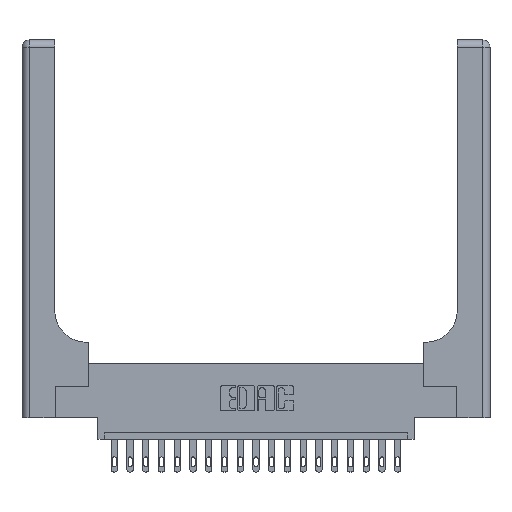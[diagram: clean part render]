
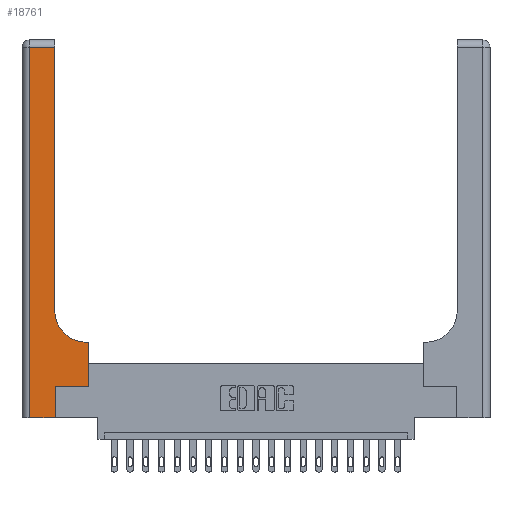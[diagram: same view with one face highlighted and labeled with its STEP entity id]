
A CAD part, top view. The second image highlights one B-rep face of the part: STEP entity #18761.
In plain terms, the highlighted planar face has unit normal (0, 0, 1).
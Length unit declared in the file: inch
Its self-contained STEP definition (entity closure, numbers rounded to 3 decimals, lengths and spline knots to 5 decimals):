
#258 = LINE ( 'NONE', #11203, #923 ) ;
#858 = CARTESIAN_POINT ( 'NONE',  ( 0.265, 0.25, 0.37 ) ) ;
#923 = VECTOR ( 'NONE', #11406, 39.37008 ) ;
#1266 = CARTESIAN_POINT ( 'NONE',  ( 0., 0., 0.37 ) ) ;
#1368 = CARTESIAN_POINT ( 'NONE',  ( 0.26, 2.94, 0.37 ) ) ;
#1375 = VECTOR ( 'NONE', #10543, 39.37008 ) ;
#1399 = LINE ( 'NONE', #14315, #11642 ) ;
#1414 = VERTEX_POINT ( 'NONE', #20177 ) ;
#1549 = VERTEX_POINT ( 'NONE', #19027 ) ;
#1613 = DIRECTION ( 'NONE',  ( 0., 1., 0. ) ) ;
#1719 = VERTEX_POINT ( 'NONE', #9852 ) ;
#1917 = CARTESIAN_POINT ( 'NONE',  ( 0.265, 0., 0.37 ) ) ;
#2539 = LINE ( 'NONE', #18473, #16022 ) ;
#2615 = VECTOR ( 'NONE', #1613, 39.37008 ) ;
#3001 = ORIENTED_EDGE ( 'NONE', *, *, #14362, .T. ) ;
#3083 = VERTEX_POINT ( 'NONE', #10987 ) ;
#3354 = EDGE_CURVE ( 'NONE', #12453, #18221, #10475, .T. ) ;
#4031 = CIRCLE ( 'NONE', #13350, 0.25 ) ;
#4135 = DIRECTION ( 'NONE',  ( -1., 0., 0. ) ) ;
#4143 = DIRECTION ( 'NONE',  ( 1., 0., 0. ) ) ;
#4725 = EDGE_CURVE ( 'NONE', #18021, #11053, #12879, .T. ) ;
#5205 = VECTOR ( 'NONE', #4135, 39.37008 ) ;
#5361 = AXIS2_PLACEMENT_3D ( 'NONE', #11034, #7587, #12482 ) ;
#7350 = CARTESIAN_POINT ( 'NONE',  ( 0., 2.94, 0.37 ) ) ;
#7587 = DIRECTION ( 'NONE',  ( 0., 0., -1. ) ) ;
#7673 = CARTESIAN_POINT ( 'NONE',  ( 0.265, 0.25, 0.37 ) ) ;
#8490 = VECTOR ( 'NONE', #19568, 39.37008 ) ;
#8946 = CARTESIAN_POINT ( 'NONE',  ( 0.265, 0., 0.37 ) ) ;
#9106 = ORIENTED_EDGE ( 'NONE', *, *, #4725, .T. ) ;
#9364 = CARTESIAN_POINT ( 'NONE',  ( 0.06, 2.94, 0.37 ) ) ;
#9852 = CARTESIAN_POINT ( 'NONE',  ( 0.06, 0., 0.37 ) ) ;
#9889 = LINE ( 'NONE', #14573, #8490 ) ;
#10297 = ORIENTED_EDGE ( 'NONE', *, *, #12374, .T. ) ;
#10475 = LINE ( 'NONE', #7350, #5205 ) ;
#10543 = DIRECTION ( 'NONE',  ( 1., 0., 0. ) ) ;
#10805 = ORIENTED_EDGE ( 'NONE', *, *, #11352, .T. ) ;
#10890 = DIRECTION ( 'NONE',  ( 0., 1., 0. ) ) ;
#10983 = VERTEX_POINT ( 'NONE', #19495 ) ;
#10987 = CARTESIAN_POINT ( 'NONE',  ( 0.51, 0.6, 0.37 ) ) ;
#11034 = CARTESIAN_POINT ( 'NONE',  ( 0., 3., 0.37 ) ) ;
#11053 = VERTEX_POINT ( 'NONE', #858 ) ;
#11203 = CARTESIAN_POINT ( 'NONE',  ( 0.528, 0.25, 0.37 ) ) ;
#11227 = LINE ( 'NONE', #7673, #15912 ) ;
#11352 = EDGE_CURVE ( 'NONE', #18221, #1719, #9889, .T. ) ;
#11406 = DIRECTION ( 'NONE',  ( 0., 1., 0. ) ) ;
#11642 = VECTOR ( 'NONE', #10890, 39.37008 ) ;
#11855 = CARTESIAN_POINT ( 'NONE',  ( 0.51, 0.85, 0.37 ) ) ;
#12374 = EDGE_CURVE ( 'NONE', #1719, #18021, #15319, .T. ) ;
#12453 = VERTEX_POINT ( 'NONE', #1368 ) ;
#12469 = DIRECTION ( 'NONE',  ( 1., 0., 0. ) ) ;
#12482 = DIRECTION ( 'NONE',  ( -1., 0., 0. ) ) ;
#12879 = LINE ( 'NONE', #1917, #2615 ) ;
#13260 = ORIENTED_EDGE ( 'NONE', *, *, #19162, .T. ) ;
#13350 = AXIS2_PLACEMENT_3D ( 'NONE', #11855, #18388, #4143 ) ;
#13750 = EDGE_CURVE ( 'NONE', #10983, #1549, #258, .T. ) ;
#13948 = EDGE_LOOP ( 'NONE', ( #20032, #19514, #10805, #10297, #9106, #3001, #17373, #16689, #13260 ) ) ;
#14315 = CARTESIAN_POINT ( 'NONE',  ( 0.26, 3., 0.37 ) ) ;
#14362 = EDGE_CURVE ( 'NONE', #11053, #10983, #11227, .T. ) ;
#14573 = CARTESIAN_POINT ( 'NONE',  ( 0.06, 3., 0.37 ) ) ;
#15319 = LINE ( 'NONE', #1266, #1375 ) ;
#15390 = PLANE ( 'NONE',  #5361 ) ;
#15912 = VECTOR ( 'NONE', #12469, 39.37008 ) ;
#16022 = VECTOR ( 'NONE', #20422, 39.37008 ) ;
#16689 = ORIENTED_EDGE ( 'NONE', *, *, #19668, .T. ) ;
#17373 = ORIENTED_EDGE ( 'NONE', *, *, #13750, .T. ) ;
#17434 = EDGE_CURVE ( 'NONE', #1414, #12453, #1399, .T. ) ;
#18021 = VERTEX_POINT ( 'NONE', #8946 ) ;
#18221 = VERTEX_POINT ( 'NONE', #9364 ) ;
#18388 = DIRECTION ( 'NONE',  ( 0., 0., -1. ) ) ;
#18473 = CARTESIAN_POINT ( 'NONE',  ( 0.26, 0.6, 0.37 ) ) ;
#18523 = FACE_OUTER_BOUND ( 'NONE', #13948, .T. ) ;
#18761 = ADVANCED_FACE ( 'NONE', ( #18523 ), #15390, .F. ) ;
#19027 = CARTESIAN_POINT ( 'NONE',  ( 0.528, 0.6, 0.37 ) ) ;
#19162 = EDGE_CURVE ( 'NONE', #3083, #1414, #4031, .T. ) ;
#19495 = CARTESIAN_POINT ( 'NONE',  ( 0.528, 0.25, 0.37 ) ) ;
#19514 = ORIENTED_EDGE ( 'NONE', *, *, #3354, .T. ) ;
#19568 = DIRECTION ( 'NONE',  ( 0., -1., 0. ) ) ;
#19668 = EDGE_CURVE ( 'NONE', #1549, #3083, #2539, .T. ) ;
#20032 = ORIENTED_EDGE ( 'NONE', *, *, #17434, .T. ) ;
#20177 = CARTESIAN_POINT ( 'NONE',  ( 0.26, 0.85, 0.37 ) ) ;
#20422 = DIRECTION ( 'NONE',  ( -1., 0., 0. ) ) ;
